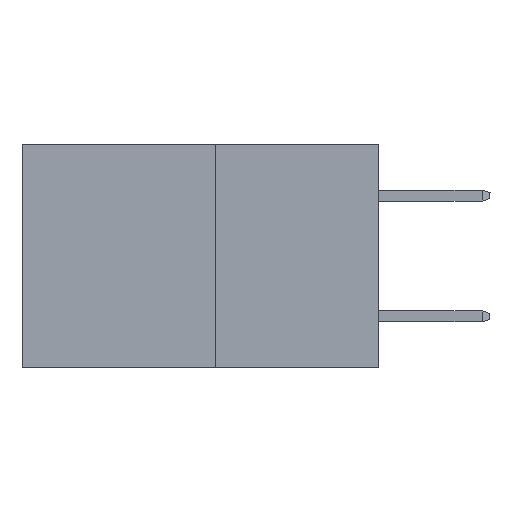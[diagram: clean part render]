
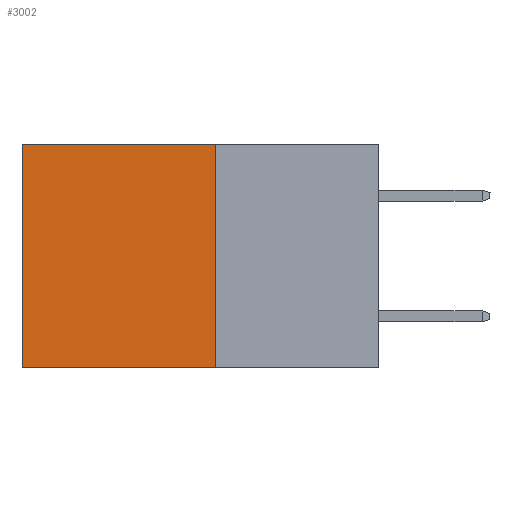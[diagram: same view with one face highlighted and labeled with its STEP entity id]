
A CAD part, left-side view. The second image highlights one B-rep face of the part: STEP entity #3002.
In plain terms, the highlighted planar face has unit normal (-1, 0, 0).
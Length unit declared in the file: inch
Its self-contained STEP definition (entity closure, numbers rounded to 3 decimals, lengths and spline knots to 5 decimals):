
#45 = VERTEX_POINT ( 'NONE', #803 ) ;
#639 = VECTOR ( 'NONE', #11384, 39.37008 ) ;
#803 = CARTESIAN_POINT ( 'NONE',  ( 0.277, 0.27, -0.37 ) ) ;
#1022 = CARTESIAN_POINT ( 'NONE',  ( 0.277, 0.27, 0. ) ) ;
#2156 = ORIENTED_EDGE ( 'NONE', *, *, #9478, .T. ) ;
#2183 = VECTOR ( 'NONE', #2905, 39.37008 ) ;
#2905 = DIRECTION ( 'NONE',  ( 0., 1., 0. ) ) ;
#3002 = ADVANCED_FACE ( 'NONE', ( #5294 ), #6550, .F. ) ;
#3451 = VERTEX_POINT ( 'NONE', #4306 ) ;
#3519 = EDGE_LOOP ( 'NONE', ( #2156, #9682, #9801, #9267 ) ) ;
#3933 = VERTEX_POINT ( 'NONE', #10835 ) ;
#4098 = EDGE_CURVE ( 'NONE', #9494, #45, #6198, .T. ) ;
#4190 = CARTESIAN_POINT ( 'NONE',  ( 0.277, 0.27, 0. ) ) ;
#4306 = CARTESIAN_POINT ( 'NONE',  ( 0.277, 0.59, -0.37 ) ) ;
#4667 = DIRECTION ( 'NONE',  ( 1., 0., 0. ) ) ;
#5294 = FACE_OUTER_BOUND ( 'NONE', #3519, .T. ) ;
#5432 = EDGE_CURVE ( 'NONE', #9494, #3933, #9930, .T. ) ;
#6198 = LINE ( 'NONE', #11725, #8869 ) ;
#6550 = PLANE ( 'NONE',  #10493 ) ;
#7098 = DIRECTION ( 'NONE',  ( 0., 0., -1. ) ) ;
#7232 = DIRECTION ( 'NONE',  ( 0., 0., -1. ) ) ;
#7432 = LINE ( 'NONE', #9914, #11941 ) ;
#8164 = DIRECTION ( 'NONE',  ( 0., 1., 0. ) ) ;
#8869 = VECTOR ( 'NONE', #7232, 39.37008 ) ;
#9267 = ORIENTED_EDGE ( 'NONE', *, *, #5432, .T. ) ;
#9478 = EDGE_CURVE ( 'NONE', #3933, #3451, #10676, .T. ) ;
#9494 = VERTEX_POINT ( 'NONE', #1022 ) ;
#9682 = ORIENTED_EDGE ( 'NONE', *, *, #10428, .F. ) ;
#9801 = ORIENTED_EDGE ( 'NONE', *, *, #4098, .F. ) ;
#9914 = CARTESIAN_POINT ( 'NONE',  ( 0.277, 0.27, -0.37 ) ) ;
#9930 = LINE ( 'NONE', #4190, #2183 ) ;
#10428 = EDGE_CURVE ( 'NONE', #45, #3451, #7432, .T. ) ;
#10465 = CARTESIAN_POINT ( 'NONE',  ( 0.277, 0.59, -0.37 ) ) ;
#10481 = CARTESIAN_POINT ( 'NONE',  ( 0.277, 0.27, -0.37 ) ) ;
#10493 = AXIS2_PLACEMENT_3D ( 'NONE', #10481, #4667, #7098 ) ;
#10676 = LINE ( 'NONE', #10465, #639 ) ;
#10835 = CARTESIAN_POINT ( 'NONE',  ( 0.277, 0.59, 0. ) ) ;
#11384 = DIRECTION ( 'NONE',  ( 0., 0., -1. ) ) ;
#11725 = CARTESIAN_POINT ( 'NONE',  ( 0.277, 0.27, -0.37 ) ) ;
#11941 = VECTOR ( 'NONE', #8164, 39.37008 ) ;
